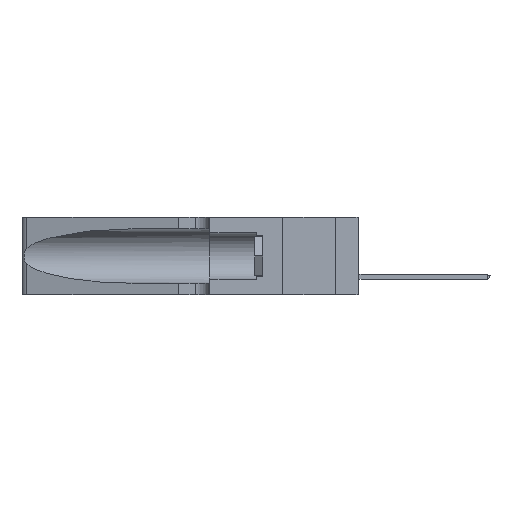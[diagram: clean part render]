
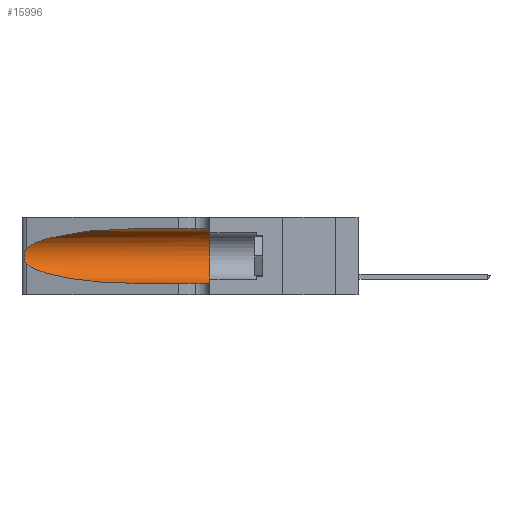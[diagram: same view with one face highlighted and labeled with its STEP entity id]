
A CAD part, left-side view. The second image highlights one B-rep face of the part: STEP entity #15996.
In plain terms, the highlighted cylindrical face has radius 3.308 mm (diameter 6.617 mm), a partial arc.
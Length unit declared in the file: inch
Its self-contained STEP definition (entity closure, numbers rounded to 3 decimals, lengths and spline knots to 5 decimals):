
#506 = CARTESIAN_POINT ( 'NONE',  ( 0.1305, 1.61858, 0.185 ) ) ;
#729 = CARTESIAN_POINT ( 'NONE',  ( 0.26075, 1.23896, 0.178 ) ) ;
#872 = LINE ( 'NONE', #4750, #31362 ) ;
#2136 = CYLINDRICAL_SURFACE ( 'NONE', #5976, 0.13025 ) ;
#4750 = CARTESIAN_POINT ( 'NONE',  ( 0.1305, 1.61858, 0.05475 ) ) ;
#5976 = AXIS2_PLACEMENT_3D ( 'NONE', #506, #17897, #34500 ) ;
#6278 = CARTESIAN_POINT ( 'NONE',  ( 0.25555, 1.22993, 0.14849 ) ) ;
#6567 = ORIENTED_EDGE ( 'NONE', *, *, #17797, .F. ) ;
#7433 = CARTESIAN_POINT ( 'NONE',  ( 0.25487, 1.22718, 0.22369 ) ) ;
#7671 = CARTESIAN_POINT ( 'NONE',  ( 0.25487, 1.22718, 0.22369 ) ) ;
#8025 = CIRCLE ( 'NONE', #29015, 0.13025 ) ;
#9343 = CARTESIAN_POINT ( 'NONE',  ( 0.18966, 0.96281, 0.05475 ) ) ;
#9390 = CARTESIAN_POINT ( 'NONE',  ( 0.25854, 1.2359, 0.20912 ) ) ;
#9720 = FACE_OUTER_BOUND ( 'NONE', #31495, .T. ) ;
#10095 = B_SPLINE_CURVE_WITH_KNOTS ( 'NONE', 3,
 ( #23662, #18100, #20972, #26396, #9390, #14791, #34722, #729, #17628, #35214, #20483, #23529, #6278, #32254 ),
 .UNSPECIFIED., .F., .F.,
 ( 4, 2, 2, 2, 2, 2, 4 ),
 ( 0., 0.00027, 0.00053, 0.00107, 0.0016, 0.00187, 0.00214 ),
 .UNSPECIFIED. ) ;
#10399 = VERTEX_POINT ( 'NONE', #34289 ) ;
#10529 = CARTESIAN_POINT ( 'NONE',  ( 0.18966, 0.96281, 0.31525 ) ) ;
#10575 = VERTEX_POINT ( 'NONE', #32444 ) ;
#11131 = CARTESIAN_POINT ( 'NONE',  ( 0.1305, 0.72297, 0.31525 ) ) ;
#11183 = ORIENTED_EDGE ( 'NONE', *, *, #22926, .F. ) ;
#11523 = VERTEX_POINT ( 'NONE', #30361 ) ;
#13892 = LINE ( 'NONE', #14594, #28621 ) ;
#14484 = DIRECTION ( 'NONE',  ( 0., -1., 0. ) ) ;
#14594 = CARTESIAN_POINT ( 'NONE',  ( 0.1305, 1.61858, 0.31525 ) ) ;
#14791 = CARTESIAN_POINT ( 'NONE',  ( 0.26018, 1.23835, 0.19895 ) ) ;
#15996 = ADVANCED_FACE ( 'NONE', ( #9720 ), #2136, .F. ) ;
#17223 = ORIENTED_EDGE ( 'NONE', *, *, #33737, .T. ) ;
#17233 =( BOUNDED_CURVE ( )  B_SPLINE_CURVE ( 3, ( #17834, #26470, #9343, #29347 ),
 .UNSPECIFIED., .F., .F. ) 
 B_SPLINE_CURVE_WITH_KNOTS ( ( 4, 4 ),
 ( 3.44316, 4.71239 ),
 .UNSPECIFIED. ) 
 CURVE ( )  GEOMETRIC_REPRESENTATION_ITEM ( )  RATIONAL_B_SPLINE_CURVE ( ( 1., 0.87, 0.87, 1. ) ) 
 REPRESENTATION_ITEM ( '' )  );
#17408 = VERTEX_POINT ( 'NONE', #20937 ) ;
#17628 = CARTESIAN_POINT ( 'NONE',  ( 0.26017, 1.23833, 0.17102 ) ) ;
#17797 = EDGE_CURVE ( 'NONE', #11523, #10575, #8025, .T. ) ;
#17834 = CARTESIAN_POINT ( 'NONE',  ( 0.25487, 1.22718, 0.14631 ) ) ;
#17897 = DIRECTION ( 'NONE',  ( 0., -1., 0. ) ) ;
#18100 = CARTESIAN_POINT ( 'NONE',  ( 0.25555, 1.22994, 0.2215 ) ) ;
#20483 = CARTESIAN_POINT ( 'NONE',  ( 0.25789, 1.23486, 0.15765 ) ) ;
#20937 = CARTESIAN_POINT ( 'NONE',  ( 0.1305, 0.72297, 0.05475 ) ) ;
#20972 = CARTESIAN_POINT ( 'NONE',  ( 0.25639, 1.23184, 0.21858 ) ) ;
#20994 = CARTESIAN_POINT ( 'NONE',  ( 0.1305, 0.72297, 0.31525 ) ) ;
#21206 = ORIENTED_EDGE ( 'NONE', *, *, #34156, .T. ) ;
#22926 = EDGE_CURVE ( 'NONE', #24081, #11523, #13892, .T. ) ;
#23529 = CARTESIAN_POINT ( 'NONE',  ( 0.25639, 1.23186, 0.15144 ) ) ;
#23662 = CARTESIAN_POINT ( 'NONE',  ( 0.25487, 1.22718, 0.22369 ) ) ;
#24081 = VERTEX_POINT ( 'NONE', #11131 ) ;
#25125 = VERTEX_POINT ( 'NONE', #7433 ) ;
#26396 = CARTESIAN_POINT ( 'NONE',  ( 0.25787, 1.23484, 0.2124 ) ) ;
#26470 = CARTESIAN_POINT ( 'NONE',  ( 0.2373, 1.15595, 0.08982 ) ) ;
#28621 = VECTOR ( 'NONE', #14484, 39.37008 ) ;
#28847 = DIRECTION ( 'NONE',  ( 0., 1., 0. ) ) ;
#29015 = AXIS2_PLACEMENT_3D ( 'NONE', #36955, #28847, #31864 ) ;
#29347 = CARTESIAN_POINT ( 'NONE',  ( 0.1305, 0.72297, 0.05475 ) ) ;
#30361 = CARTESIAN_POINT ( 'NONE',  ( 0.1305, 0.35, 0.31525 ) ) ;
#30519 = DIRECTION ( 'NONE',  ( 0., -1., 0. ) ) ;
#31362 = VECTOR ( 'NONE', #30519, 39.37008 ) ;
#31495 = EDGE_LOOP ( 'NONE', ( #35182, #36244, #21206, #17223, #6567, #11183 ) ) ;
#31864 = DIRECTION ( 'NONE',  ( 0., 0., 1. ) ) ;
#32254 = CARTESIAN_POINT ( 'NONE',  ( 0.25487, 1.22718, 0.14631 ) ) ;
#32444 = CARTESIAN_POINT ( 'NONE',  ( 0.1305, 0.35, 0.05475 ) ) ;
#32988 = EDGE_CURVE ( 'NONE', #24081, #25125, #34847, .T. ) ;
#33257 = CARTESIAN_POINT ( 'NONE',  ( 0.2373, 1.15595, 0.28018 ) ) ;
#33378 = EDGE_CURVE ( 'NONE', #25125, #10399, #10095, .T. ) ;
#33737 = EDGE_CURVE ( 'NONE', #17408, #10575, #872, .T. ) ;
#34156 = EDGE_CURVE ( 'NONE', #10399, #17408, #17233, .T. ) ;
#34289 = CARTESIAN_POINT ( 'NONE',  ( 0.25487, 1.22718, 0.14631 ) ) ;
#34500 = DIRECTION ( 'NONE',  ( 0., 0., -1. ) ) ;
#34722 = CARTESIAN_POINT ( 'NONE',  ( 0.26075, 1.23896, 0.19203 ) ) ;
#34847 =( BOUNDED_CURVE ( )  B_SPLINE_CURVE ( 3, ( #20994, #10529, #33257, #7671 ),
 .UNSPECIFIED., .F., .F. ) 
 B_SPLINE_CURVE_WITH_KNOTS ( ( 4, 4 ),
 ( 1.5708, 2.84003 ),
 .UNSPECIFIED. ) 
 CURVE ( )  GEOMETRIC_REPRESENTATION_ITEM ( )  RATIONAL_B_SPLINE_CURVE ( ( 1., 0.87, 0.87, 1. ) ) 
 REPRESENTATION_ITEM ( '' )  );
#35182 = ORIENTED_EDGE ( 'NONE', *, *, #32988, .T. ) ;
#35214 = CARTESIAN_POINT ( 'NONE',  ( 0.25856, 1.23593, 0.16098 ) ) ;
#36244 = ORIENTED_EDGE ( 'NONE', *, *, #33378, .T. ) ;
#36955 = CARTESIAN_POINT ( 'NONE',  ( 0.1305, 0.35, 0.185 ) ) ;
